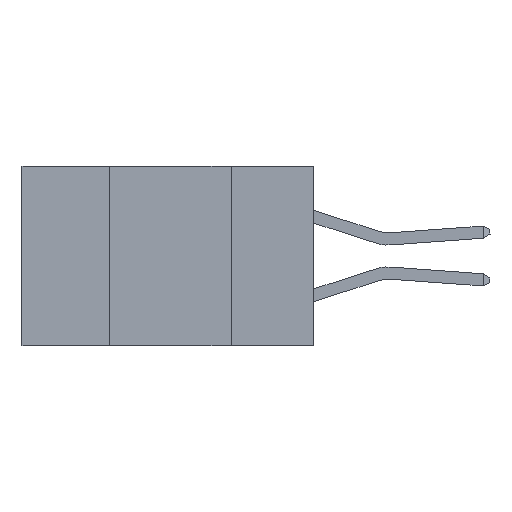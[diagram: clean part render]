
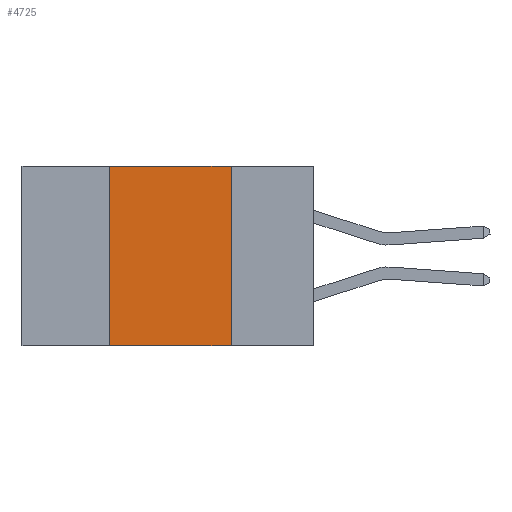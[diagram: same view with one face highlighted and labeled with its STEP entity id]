
A CAD part, left-side view. The second image highlights one B-rep face of the part: STEP entity #4725.
In plain terms, the highlighted planar face has unit normal (-1, 0, 0).
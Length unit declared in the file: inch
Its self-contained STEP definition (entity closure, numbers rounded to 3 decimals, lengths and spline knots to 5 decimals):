
#2031 = EDGE_CURVE ( 'NONE', #31723, #16773, #15816, .T. ) ;
#2778 = VERTEX_POINT ( 'NONE', #20726 ) ;
#2783 = ORIENTED_EDGE ( 'NONE', *, *, #32242, .F. ) ;
#3641 = VERTEX_POINT ( 'NONE', #9061 ) ;
#3818 = CARTESIAN_POINT ( 'NONE',  ( 0., 0.17, 0. ) ) ;
#3964 = VECTOR ( 'NONE', #12129, 39.37008 ) ;
#4719 = VECTOR ( 'NONE', #12711, 39.37008 ) ;
#4725 = ADVANCED_FACE ( 'NONE', ( #4814 ), #23328, .F. ) ;
#4814 = FACE_OUTER_BOUND ( 'NONE', #26997, .T. ) ;
#6258 = DIRECTION ( 'NONE',  ( 0., 0., 1. ) ) ;
#7231 = DIRECTION ( 'NONE',  ( 0., 0., -1. ) ) ;
#8351 = CARTESIAN_POINT ( 'NONE',  ( 0., 0.17, 0. ) ) ;
#9061 = CARTESIAN_POINT ( 'NONE',  ( 0., 0.17, -0.37 ) ) ;
#9853 = EDGE_CURVE ( 'NONE', #16773, #3641, #23786, .T. ) ;
#10510 = DIRECTION ( 'NONE',  ( 1., 0., 0. ) ) ;
#11027 = CARTESIAN_POINT ( 'NONE',  ( 0., 0.42, 0. ) ) ;
#12129 = DIRECTION ( 'NONE',  ( 0., -1., 0. ) ) ;
#12406 = VECTOR ( 'NONE', #21362, 39.37008 ) ;
#12711 = DIRECTION ( 'NONE',  ( 0., -1., 0. ) ) ;
#12861 = AXIS2_PLACEMENT_3D ( 'NONE', #20734, #10510, #7231 ) ;
#15816 = LINE ( 'NONE', #20672, #4719 ) ;
#16773 = VERTEX_POINT ( 'NONE', #3818 ) ;
#17143 = LINE ( 'NONE', #22697, #3964 ) ;
#18236 = EDGE_CURVE ( 'NONE', #2778, #3641, #17143, .T. ) ;
#18521 = VECTOR ( 'NONE', #6258, 39.37008 ) ;
#19254 = CARTESIAN_POINT ( 'NONE',  ( 0., 0.42, 0. ) ) ;
#20672 = CARTESIAN_POINT ( 'NONE',  ( 0., 0.6, 0. ) ) ;
#20726 = CARTESIAN_POINT ( 'NONE',  ( 0., 0.42, -0.37 ) ) ;
#20734 = CARTESIAN_POINT ( 'NONE',  ( 0., 0.6, 0. ) ) ;
#21362 = DIRECTION ( 'NONE',  ( 0., 0., -1. ) ) ;
#22697 = CARTESIAN_POINT ( 'NONE',  ( 0., 0.6, -0.37 ) ) ;
#23328 = PLANE ( 'NONE',  #12861 ) ;
#23786 = LINE ( 'NONE', #8351, #12406 ) ;
#26997 = EDGE_LOOP ( 'NONE', ( #31134, #29920, #2783, #31436 ) ) ;
#27739 = LINE ( 'NONE', #19254, #18521 ) ;
#29920 = ORIENTED_EDGE ( 'NONE', *, *, #2031, .F. ) ;
#31134 = ORIENTED_EDGE ( 'NONE', *, *, #9853, .F. ) ;
#31436 = ORIENTED_EDGE ( 'NONE', *, *, #18236, .T. ) ;
#31723 = VERTEX_POINT ( 'NONE', #11027 ) ;
#32242 = EDGE_CURVE ( 'NONE', #2778, #31723, #27739, .T. ) ;
